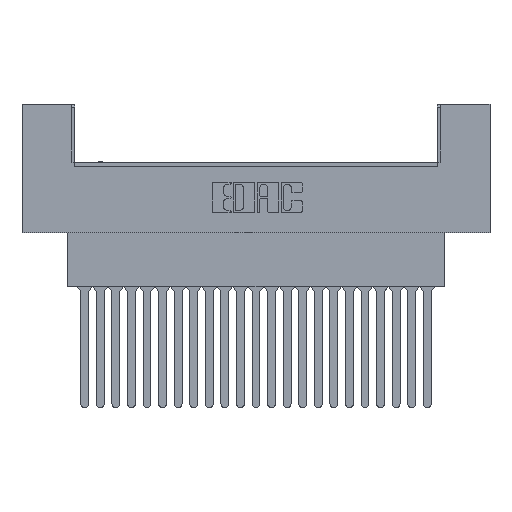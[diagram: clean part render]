
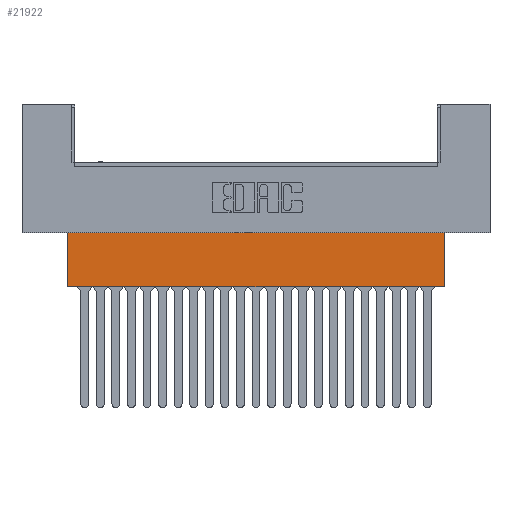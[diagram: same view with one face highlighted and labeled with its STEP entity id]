
A CAD part, top view. The second image highlights one B-rep face of the part: STEP entity #21922.
In plain terms, the highlighted planar face has unit normal (0, 0, 1).
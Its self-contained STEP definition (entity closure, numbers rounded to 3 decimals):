
#507 = AXIS2_PLACEMENT_3D ( 'NONE', #15160, #22135, #19615 ) ;
#1122 = CARTESIAN_POINT ( 'NONE',  ( 7.468, -8.814, -3.962 ) ) ;
#2235 = DIRECTION ( 'NONE',  ( 0., -1., 0. ) ) ;
#2340 = CARTESIAN_POINT ( 'NONE',  ( 68.885, -8.814, -3.962 ) ) ;
#2929 = ORIENTED_EDGE ( 'NONE', *, *, #8011, .T. ) ;
#3479 = CARTESIAN_POINT ( 'NONE',  ( 68.885, -8.814, -3.962 ) ) ;
#3599 = EDGE_LOOP ( 'NONE', ( #12931, #26534, #2929, #9605 ) ) ;
#3603 = FACE_OUTER_BOUND ( 'NONE', #3599, .T. ) ;
#4185 = VERTEX_POINT ( 'NONE', #20342 ) ;
#7860 = DIRECTION ( 'NONE',  ( 0., 1., 0. ) ) ;
#8011 = EDGE_CURVE ( 'NONE', #4185, #20275, #17871, .T. ) ;
#8832 = VECTOR ( 'NONE', #18061, 1000. ) ;
#9605 = ORIENTED_EDGE ( 'NONE', *, *, #24666, .F. ) ;
#10241 = CARTESIAN_POINT ( 'NONE',  ( 76.352, -8.814, -3.962 ) ) ;
#10977 = EDGE_CURVE ( 'NONE', #23978, #14366, #11691, .T. ) ;
#11691 = LINE ( 'NONE', #10241, #26861 ) ;
#11712 = LINE ( 'NONE', #1122, #27255 ) ;
#12374 = EDGE_CURVE ( 'NONE', #4185, #23978, #17391, .T. ) ;
#12931 = ORIENTED_EDGE ( 'NONE', *, *, #10977, .F. ) ;
#14107 = VECTOR ( 'NONE', #2235, 1000. ) ;
#14366 = VERTEX_POINT ( 'NONE', #26052 ) ;
#14962 = PLANE ( 'NONE',  #507 ) ;
#15160 = CARTESIAN_POINT ( 'NONE',  ( 76.352, 0., -3.962 ) ) ;
#17391 = LINE ( 'NONE', #2340, #14107 ) ;
#17668 = CARTESIAN_POINT ( 'NONE',  ( 7.468, 0., -3.962 ) ) ;
#17871 = LINE ( 'NONE', #20165, #8832 ) ;
#18061 = DIRECTION ( 'NONE',  ( -1., 0., 0. ) ) ;
#19615 = DIRECTION ( 'NONE',  ( 0., 1., 0. ) ) ;
#20165 = CARTESIAN_POINT ( 'NONE',  ( 76.352, 0., -3.962 ) ) ;
#20275 = VERTEX_POINT ( 'NONE', #17668 ) ;
#20342 = CARTESIAN_POINT ( 'NONE',  ( 68.885, 0., -3.962 ) ) ;
#21922 = ADVANCED_FACE ( 'NONE', ( #3603 ), #14962, .F. ) ;
#22135 = DIRECTION ( 'NONE',  ( 0., 0., -1. ) ) ;
#23978 = VERTEX_POINT ( 'NONE', #3479 ) ;
#24666 = EDGE_CURVE ( 'NONE', #14366, #20275, #11712, .T. ) ;
#26052 = CARTESIAN_POINT ( 'NONE',  ( 7.468, -8.814, -3.962 ) ) ;
#26468 = DIRECTION ( 'NONE',  ( -1., 0., 0. ) ) ;
#26534 = ORIENTED_EDGE ( 'NONE', *, *, #12374, .F. ) ;
#26861 = VECTOR ( 'NONE', #26468, 1000. ) ;
#27255 = VECTOR ( 'NONE', #7860, 1000. ) ;
